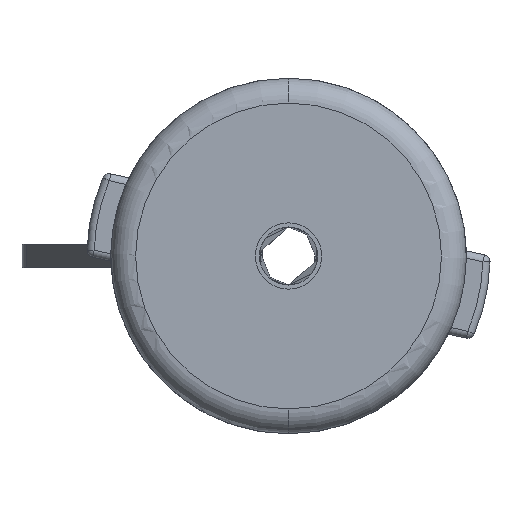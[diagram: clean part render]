
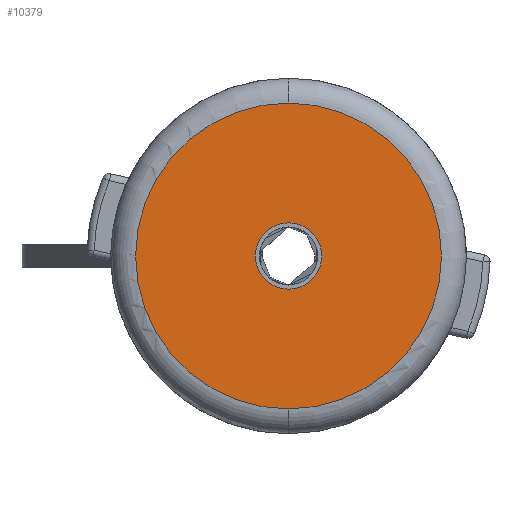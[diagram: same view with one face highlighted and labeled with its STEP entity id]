
A CAD part, front view. The second image highlights one B-rep face of the part: STEP entity #10379.
In plain terms, the highlighted planar face has unit normal (0, -1, 0).
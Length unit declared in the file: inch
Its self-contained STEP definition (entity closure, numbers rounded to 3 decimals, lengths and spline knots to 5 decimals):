
#988 = CARTESIAN_POINT ( 'NONE',  ( 0., 0., 0. ) ) ;
#1809 = EDGE_CURVE ( 'NONE', #12325, #10427, #3199, .T. ) ;
#1875 = AXIS2_PLACEMENT_3D ( 'NONE', #9452, #3475, #10458 ) ;
#1997 = DIRECTION ( 'NONE',  ( 0., 0., 1. ) ) ;
#2115 = DIRECTION ( 'NONE',  ( 0., 1., 0. ) ) ;
#2350 = CARTESIAN_POINT ( 'NONE',  ( 0., 0., 0. ) ) ;
#3199 = CIRCLE ( 'NONE', #9342, 0.14 ) ;
#3339 = DIRECTION ( 'NONE',  ( 0., -1., 0. ) ) ;
#3475 = DIRECTION ( 'NONE',  ( 0., -1., 0. ) ) ;
#3903 = EDGE_CURVE ( 'NONE', #9001, #4242, #10367, .T. ) ;
#4242 = VERTEX_POINT ( 'NONE', #8012 ) ;
#4392 = CIRCLE ( 'NONE', #1875, 0.645 ) ;
#4931 = DIRECTION ( 'NONE',  ( 0., -1., 0. ) ) ;
#5059 = CARTESIAN_POINT ( 'NONE',  ( 0., 0., 0.645 ) ) ;
#5673 = EDGE_CURVE ( 'NONE', #10427, #12325, #10857, .T. ) ;
#5942 = FACE_OUTER_BOUND ( 'NONE', #7170, .T. ) ;
#6143 = AXIS2_PLACEMENT_3D ( 'NONE', #2350, #3339, #10313 ) ;
#6989 = ORIENTED_EDGE ( 'NONE', *, *, #3903, .T. ) ;
#7170 = EDGE_LOOP ( 'NONE', ( #12671, #6989 ) ) ;
#7966 = DIRECTION ( 'NONE',  ( 0., 1., 0. ) ) ;
#8012 = CARTESIAN_POINT ( 'NONE',  ( 0., 0., -0.645 ) ) ;
#8087 = CARTESIAN_POINT ( 'NONE',  ( 0., 0., 0. ) ) ;
#8299 = FACE_BOUND ( 'NONE', #10087, .T. ) ;
#8319 = PLANE ( 'NONE',  #6143 ) ;
#9001 = VERTEX_POINT ( 'NONE', #5059 ) ;
#9077 = DIRECTION ( 'NONE',  ( 0., 0., 1. ) ) ;
#9170 = EDGE_CURVE ( 'NONE', #4242, #9001, #4392, .T. ) ;
#9342 = AXIS2_PLACEMENT_3D ( 'NONE', #988, #7966, #1997 ) ;
#9452 = CARTESIAN_POINT ( 'NONE',  ( 0., 0., 0. ) ) ;
#9533 = CARTESIAN_POINT ( 'NONE',  ( 0., 0., -0.14 ) ) ;
#9696 = AXIS2_PLACEMENT_3D ( 'NONE', #10928, #4931, #11944 ) ;
#10087 = EDGE_LOOP ( 'NONE', ( #12347, #12939 ) ) ;
#10313 = DIRECTION ( 'NONE',  ( 0., 0., -1. ) ) ;
#10359 = CARTESIAN_POINT ( 'NONE',  ( 0., 0., 0.14 ) ) ;
#10367 = CIRCLE ( 'NONE', #9696, 0.645 ) ;
#10379 = ADVANCED_FACE ( 'NONE', ( #5942, #8299 ), #8319, .T. ) ;
#10427 = VERTEX_POINT ( 'NONE', #10359 ) ;
#10458 = DIRECTION ( 'NONE',  ( 0., 0., -1. ) ) ;
#10857 = CIRCLE ( 'NONE', #11643, 0.14 ) ;
#10928 = CARTESIAN_POINT ( 'NONE',  ( 0., 0., 0. ) ) ;
#11643 = AXIS2_PLACEMENT_3D ( 'NONE', #8087, #2115, #9077 ) ;
#11944 = DIRECTION ( 'NONE',  ( 0., 0., -1. ) ) ;
#12325 = VERTEX_POINT ( 'NONE', #9533 ) ;
#12347 = ORIENTED_EDGE ( 'NONE', *, *, #1809, .T. ) ;
#12671 = ORIENTED_EDGE ( 'NONE', *, *, #9170, .T. ) ;
#12939 = ORIENTED_EDGE ( 'NONE', *, *, #5673, .T. ) ;
